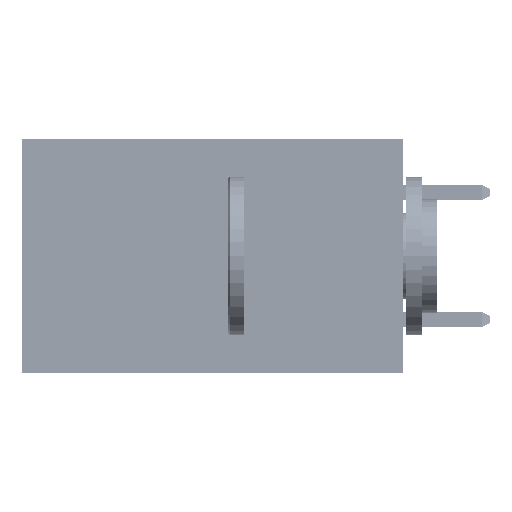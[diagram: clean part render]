
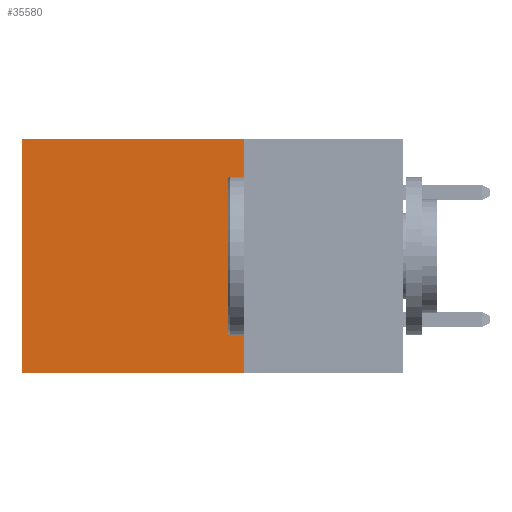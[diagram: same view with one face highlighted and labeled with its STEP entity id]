
A CAD part, left-side view. The second image highlights one B-rep face of the part: STEP entity #35580.
In plain terms, the highlighted planar face has unit normal (-1, 0, 0).
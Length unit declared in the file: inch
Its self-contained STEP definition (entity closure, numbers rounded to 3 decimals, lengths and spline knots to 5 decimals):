
#1662 = DIRECTION ( 'NONE',  ( 1., 0., 0. ) ) ;
#6464 = AXIS2_PLACEMENT_3D ( 'NONE', #24468, #1662, #28303 ) ;
#6790 = CARTESIAN_POINT ( 'NONE',  ( 0.2875, 0.6, -0.37 ) ) ;
#6792 = EDGE_CURVE ( 'NONE', #39201, #38772, #32665, .T. ) ;
#9139 = CARTESIAN_POINT ( 'NONE',  ( 0.2875, 0.6, 0. ) ) ;
#9160 = DIRECTION ( 'NONE',  ( 0., 1., 0. ) ) ;
#11105 = EDGE_LOOP ( 'NONE', ( #31268, #22848, #13529, #42721 ) ) ;
#12477 = LINE ( 'NONE', #31899, #43984 ) ;
#13529 = ORIENTED_EDGE ( 'NONE', *, *, #23173, .F. ) ;
#15162 = VECTOR ( 'NONE', #23309, 39.37008 ) ;
#15350 = VERTEX_POINT ( 'NONE', #16610 ) ;
#16610 = CARTESIAN_POINT ( 'NONE',  ( 0.2875, 0.25, -0.37 ) ) ;
#18092 = CARTESIAN_POINT ( 'NONE',  ( 0.2875, 0.25, 0. ) ) ;
#21459 = CARTESIAN_POINT ( 'NONE',  ( 0.2875, 0.25, 0. ) ) ;
#22848 = ORIENTED_EDGE ( 'NONE', *, *, #36957, .F. ) ;
#23173 = EDGE_CURVE ( 'NONE', #39201, #15350, #25269, .T. ) ;
#23309 = DIRECTION ( 'NONE',  ( 0., 0., -1. ) ) ;
#24296 = PLANE ( 'NONE',  #6464 ) ;
#24468 = CARTESIAN_POINT ( 'NONE',  ( 0.2875, 0.25, 0. ) ) ;
#24815 = CARTESIAN_POINT ( 'NONE',  ( 0.2875, 0.6, 0. ) ) ;
#25269 = LINE ( 'NONE', #26984, #15162 ) ;
#26984 = CARTESIAN_POINT ( 'NONE',  ( 0.2875, 0.25, 0. ) ) ;
#28303 = DIRECTION ( 'NONE',  ( 0., 0., -1. ) ) ;
#28627 = DIRECTION ( 'NONE',  ( 0., 0., -1. ) ) ;
#31268 = ORIENTED_EDGE ( 'NONE', *, *, #38123, .T. ) ;
#31899 = CARTESIAN_POINT ( 'NONE',  ( 0.2875, 0.25, -0.37 ) ) ;
#32665 = LINE ( 'NONE', #18092, #42783 ) ;
#33145 = DIRECTION ( 'NONE',  ( 0., 1., 0. ) ) ;
#34327 = VECTOR ( 'NONE', #28627, 39.37008 ) ;
#35580 = ADVANCED_FACE ( 'NONE', ( #41747 ), #24296, .F. ) ;
#36957 = EDGE_CURVE ( 'NONE', #15350, #42732, #12477, .T. ) ;
#38123 = EDGE_CURVE ( 'NONE', #38772, #42732, #45646, .T. ) ;
#38772 = VERTEX_POINT ( 'NONE', #9139 ) ;
#39201 = VERTEX_POINT ( 'NONE', #21459 ) ;
#41747 = FACE_OUTER_BOUND ( 'NONE', #11105, .T. ) ;
#42721 = ORIENTED_EDGE ( 'NONE', *, *, #6792, .T. ) ;
#42732 = VERTEX_POINT ( 'NONE', #6790 ) ;
#42783 = VECTOR ( 'NONE', #33145, 39.37008 ) ;
#43984 = VECTOR ( 'NONE', #9160, 39.37008 ) ;
#45646 = LINE ( 'NONE', #24815, #34327 ) ;
